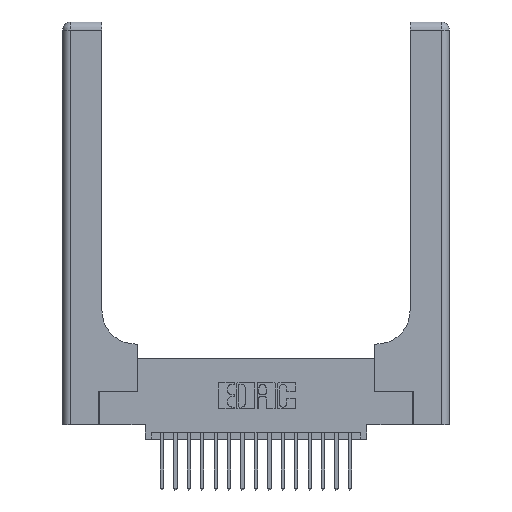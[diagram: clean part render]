
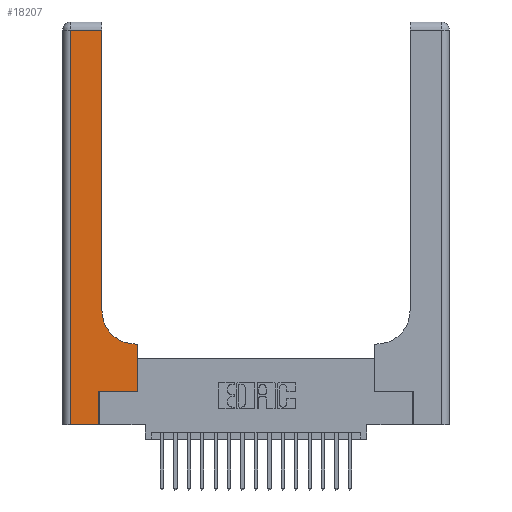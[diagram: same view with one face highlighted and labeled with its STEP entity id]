
A CAD part, top view. The second image highlights one B-rep face of the part: STEP entity #18207.
In plain terms, the highlighted planar face has unit normal (0, 0, 1).
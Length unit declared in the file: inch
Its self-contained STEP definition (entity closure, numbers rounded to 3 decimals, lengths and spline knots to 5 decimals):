
#169 = VERTEX_POINT ( 'NONE', #9061 ) ;
#414 = VERTEX_POINT ( 'NONE', #15769 ) ;
#430 = LINE ( 'NONE', #3612, #12855 ) ;
#653 = DIRECTION ( 'NONE',  ( 0., 0., -1. ) ) ;
#1201 = LINE ( 'NONE', #4646, #9333 ) ;
#1521 = ORIENTED_EDGE ( 'NONE', *, *, #2426, .T. ) ;
#1605 = VECTOR ( 'NONE', #18866, 39.37008 ) ;
#2426 = EDGE_CURVE ( 'NONE', #169, #16669, #430, .T. ) ;
#2926 = VERTEX_POINT ( 'NONE', #5122 ) ;
#3598 = DIRECTION ( 'NONE',  ( 0., 1., 0. ) ) ;
#3612 = CARTESIAN_POINT ( 'NONE',  ( 0.269, 0., 0.37 ) ) ;
#3638 = VERTEX_POINT ( 'NONE', #16656 ) ;
#3659 = DIRECTION ( 'NONE',  ( -1., 0., 0. ) ) ;
#3921 = VECTOR ( 'NONE', #3659, 39.37008 ) ;
#4646 = CARTESIAN_POINT ( 'NONE',  ( 0.2915, 3., 0.37 ) ) ;
#4700 = CARTESIAN_POINT ( 'NONE',  ( 0.06, 3., 0.37 ) ) ;
#5002 = AXIS2_PLACEMENT_3D ( 'NONE', #10391, #653, #11996 ) ;
#5057 = DIRECTION ( 'NONE',  ( 0., 0., -1. ) ) ;
#5075 = VERTEX_POINT ( 'NONE', #17010 ) ;
#5113 = CARTESIAN_POINT ( 'NONE',  ( 0.269, 0.25, 0.37 ) ) ;
#5122 = CARTESIAN_POINT ( 'NONE',  ( 0.2915, 2.94, 0.37 ) ) ;
#5395 = CARTESIAN_POINT ( 'NONE',  ( 0.06, 2.94, 0.37 ) ) ;
#5691 = ORIENTED_EDGE ( 'NONE', *, *, #17083, .T. ) ;
#5757 = CARTESIAN_POINT ( 'NONE',  ( 0.2915, 0.85, 0.37 ) ) ;
#5793 = VERTEX_POINT ( 'NONE', #5395 ) ;
#6032 = LINE ( 'NONE', #13645, #9791 ) ;
#6121 = EDGE_CURVE ( 'NONE', #8810, #2926, #1201, .T. ) ;
#6759 = DIRECTION ( 'NONE',  ( 1., 0., 0. ) ) ;
#7444 = ORIENTED_EDGE ( 'NONE', *, *, #9225, .T. ) ;
#7753 = LINE ( 'NONE', #14922, #3921 ) ;
#7934 = DIRECTION ( 'NONE',  ( 0., 1., 0. ) ) ;
#8810 = VERTEX_POINT ( 'NONE', #5757 ) ;
#8847 = DIRECTION ( 'NONE',  ( 0., 1., 0. ) ) ;
#8891 = DIRECTION ( 'NONE',  ( -1., 0., 0. ) ) ;
#9032 = ORIENTED_EDGE ( 'NONE', *, *, #18008, .T. ) ;
#9061 = CARTESIAN_POINT ( 'NONE',  ( 0.269, 0., 0.37 ) ) ;
#9225 = EDGE_CURVE ( 'NONE', #5075, #10067, #7753, .T. ) ;
#9333 = VECTOR ( 'NONE', #7934, 39.37008 ) ;
#9791 = VECTOR ( 'NONE', #8847, 39.37008 ) ;
#9843 = CARTESIAN_POINT ( 'NONE',  ( 0., 3., 0.37 ) ) ;
#10067 = VERTEX_POINT ( 'NONE', #20536 ) ;
#10104 = ORIENTED_EDGE ( 'NONE', *, *, #11346, .T. ) ;
#10282 = EDGE_CURVE ( 'NONE', #16669, #3638, #15201, .T. ) ;
#10391 = CARTESIAN_POINT ( 'NONE',  ( 0.5415, 0.85, 0.37 ) ) ;
#10974 = CARTESIAN_POINT ( 'NONE',  ( 0., 0., 0.37 ) ) ;
#11346 = EDGE_CURVE ( 'NONE', #3638, #5075, #6032, .T. ) ;
#11996 = DIRECTION ( 'NONE',  ( 1., 0., 0. ) ) ;
#12116 = CARTESIAN_POINT ( 'NONE',  ( 0., 2.94, 0.37 ) ) ;
#12282 = EDGE_CURVE ( 'NONE', #5793, #414, #16006, .T. ) ;
#12660 = DIRECTION ( 'NONE',  ( 0., -1., 0. ) ) ;
#12855 = VECTOR ( 'NONE', #3598, 39.37008 ) ;
#13505 = CIRCLE ( 'NONE', #5002, 0.25 ) ;
#13645 = CARTESIAN_POINT ( 'NONE',  ( 0.5585, 0.25, 0.37 ) ) ;
#13785 = ORIENTED_EDGE ( 'NONE', *, *, #19539, .T. ) ;
#14647 = ORIENTED_EDGE ( 'NONE', *, *, #10282, .T. ) ;
#14922 = CARTESIAN_POINT ( 'NONE',  ( 0.2915, 0.6, 0.37 ) ) ;
#15201 = LINE ( 'NONE', #5113, #18871 ) ;
#15769 = CARTESIAN_POINT ( 'NONE',  ( 0.06, 0., 0.37 ) ) ;
#16006 = LINE ( 'NONE', #4700, #19180 ) ;
#16264 = DIRECTION ( 'NONE',  ( -1., 0., 0. ) ) ;
#16656 = CARTESIAN_POINT ( 'NONE',  ( 0.5585, 0.25, 0.37 ) ) ;
#16665 = CARTESIAN_POINT ( 'NONE',  ( 0.269, 0.25, 0.37 ) ) ;
#16669 = VERTEX_POINT ( 'NONE', #16665 ) ;
#16704 = AXIS2_PLACEMENT_3D ( 'NONE', #9843, #5057, #16264 ) ;
#17010 = CARTESIAN_POINT ( 'NONE',  ( 0.5585, 0.6, 0.37 ) ) ;
#17083 = EDGE_CURVE ( 'NONE', #10067, #8810, #13505, .T. ) ;
#17413 = EDGE_LOOP ( 'NONE', ( #17929, #13785, #19734, #9032, #1521, #14647, #10104, #7444, #5691 ) ) ;
#17929 = ORIENTED_EDGE ( 'NONE', *, *, #6121, .T. ) ;
#18008 = EDGE_CURVE ( 'NONE', #414, #169, #18195, .T. ) ;
#18195 = LINE ( 'NONE', #10974, #1605 ) ;
#18207 = ADVANCED_FACE ( 'NONE', ( #18899 ), #19333, .F. ) ;
#18866 = DIRECTION ( 'NONE',  ( 1., 0., 0. ) ) ;
#18871 = VECTOR ( 'NONE', #6759, 39.37008 ) ;
#18899 = FACE_OUTER_BOUND ( 'NONE', #17413, .T. ) ;
#19180 = VECTOR ( 'NONE', #12660, 39.37008 ) ;
#19333 = PLANE ( 'NONE',  #16704 ) ;
#19539 = EDGE_CURVE ( 'NONE', #2926, #5793, #20300, .T. ) ;
#19734 = ORIENTED_EDGE ( 'NONE', *, *, #12282, .T. ) ;
#19810 = VECTOR ( 'NONE', #8891, 39.37008 ) ;
#20300 = LINE ( 'NONE', #12116, #19810 ) ;
#20536 = CARTESIAN_POINT ( 'NONE',  ( 0.5415, 0.6, 0.37 ) ) ;
